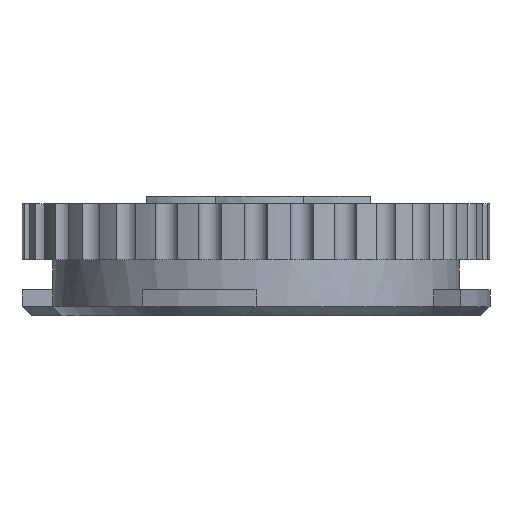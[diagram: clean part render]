
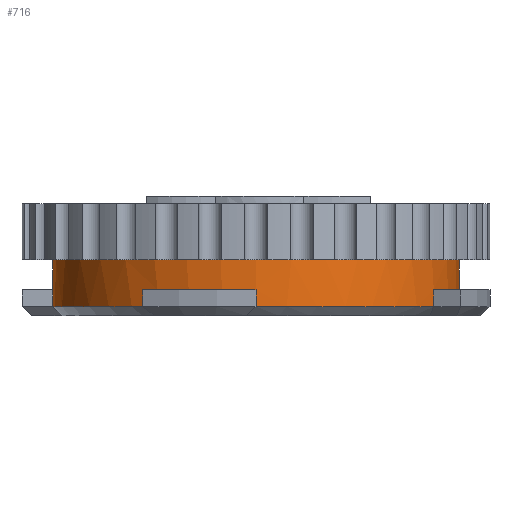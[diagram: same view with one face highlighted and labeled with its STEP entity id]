
A CAD part, front view. The second image highlights one B-rep face of the part: STEP entity #716.
In plain terms, the highlighted cylindrical face has radius 13.787 mm (diameter 27.575 mm), a partial arc.
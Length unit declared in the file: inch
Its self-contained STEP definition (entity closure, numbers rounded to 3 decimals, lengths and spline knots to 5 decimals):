
#70 = VECTOR ( 'NONE', #9266, 39.37008 ) ;
#74 = CARTESIAN_POINT ( 'NONE',  ( -0.26316, -0.47476, 0.15 ) ) ;
#172 = DIRECTION ( 'NONE',  ( 0., 0., 1. ) ) ;
#273 = EDGE_CURVE ( 'NONE', #2922, #9661, #8090, .T. ) ;
#299 = EDGE_CURVE ( 'NONE', #7053, #6835, #10244, .T. ) ;
#336 = VECTOR ( 'NONE', #3346, 39.37008 ) ;
#481 = VERTEX_POINT ( 'NONE', #3257 ) ;
#513 = LINE ( 'NONE', #5966, #7070 ) ;
#571 = DIRECTION ( 'NONE',  ( 0., 0., 1. ) ) ;
#663 = CARTESIAN_POINT ( 'NONE',  ( 0., -0.54281, 0.02461 ) ) ;
#678 = FACE_OUTER_BOUND ( 'NONE', #6350, .T. ) ;
#716 = ADVANCED_FACE ( 'NONE', ( #678 ), #5493, .T. ) ;
#2026 = DIRECTION ( 'NONE',  ( 1., 0., 0. ) ) ;
#2131 = EDGE_CURVE ( 'NONE', #2906, #481, #11769, .T. ) ;
#2173 = EDGE_CURVE ( 'NONE', #5177, #5873, #8342, .T. ) ;
#2304 = DIRECTION ( 'NONE',  ( 0., 0., -1. ) ) ;
#2452 = VECTOR ( 'NONE', #10574, 39.37008 ) ;
#2470 = AXIS2_PLACEMENT_3D ( 'NONE', #10222, #7526, #8386 ) ;
#2478 = CARTESIAN_POINT ( 'NONE',  ( -0.54281, 0., 0.15 ) ) ;
#2486 = ORIENTED_EDGE ( 'NONE', *, *, #6301, .T. ) ;
#2507 = LINE ( 'NONE', #7438, #70 ) ;
#2511 = DIRECTION ( 'NONE',  ( 0., 0., 1. ) ) ;
#2636 = DIRECTION ( 'NONE',  ( 1., 0., 0. ) ) ;
#2906 = VERTEX_POINT ( 'NONE', #7974 ) ;
#2922 = VERTEX_POINT ( 'NONE', #2478 ) ;
#3010 = ORIENTED_EDGE ( 'NONE', *, *, #2173, .T. ) ;
#3013 = AXIS2_PLACEMENT_3D ( 'NONE', #8129, #6281, #2636 ) ;
#3239 = DIRECTION ( 'NONE',  ( 0., 0., 1. ) ) ;
#3257 = CARTESIAN_POINT ( 'NONE',  ( 0.54281, 0., 0.07 ) ) ;
#3346 = DIRECTION ( 'NONE',  ( 0., 0., -1. ) ) ;
#3484 = ORIENTED_EDGE ( 'NONE', *, *, #3517, .T. ) ;
#3517 = EDGE_CURVE ( 'NONE', #4905, #8019, #4777, .T. ) ;
#4618 = VECTOR ( 'NONE', #8331, 39.37008 ) ;
#4669 = CARTESIAN_POINT ( 'NONE',  ( 0., 0., 0.02461 ) ) ;
#4703 = DIRECTION ( 'NONE',  ( 0., 0., 1. ) ) ;
#4777 = CIRCLE ( 'NONE', #10552, 0.54281 ) ;
#4895 = LINE ( 'NONE', #74, #4618 ) ;
#4905 = VERTEX_POINT ( 'NONE', #11013 ) ;
#4997 = CARTESIAN_POINT ( 'NONE',  ( -0.54281, 0., 0.07 ) ) ;
#5053 = ORIENTED_EDGE ( 'NONE', *, *, #2131, .T. ) ;
#5093 = AXIS2_PLACEMENT_3D ( 'NONE', #9756, #571, #7854 ) ;
#5177 = VERTEX_POINT ( 'NONE', #4997 ) ;
#5230 = EDGE_CURVE ( 'NONE', #6835, #2906, #513, .T. ) ;
#5493 = CYLINDRICAL_SURFACE ( 'NONE', #2470, 0.54281 ) ;
#5568 = EDGE_CURVE ( 'NONE', #5873, #7610, #11511, .T. ) ;
#5571 = AXIS2_PLACEMENT_3D ( 'NONE', #11255, #4703, #9412 ) ;
#5873 = VERTEX_POINT ( 'NONE', #7384 ) ;
#5943 = CARTESIAN_POINT ( 'NONE',  ( -0.54281, 0., 0.15 ) ) ;
#5960 = CARTESIAN_POINT ( 'NONE',  ( -0.54281, 0., 0.15 ) ) ;
#5966 = CARTESIAN_POINT ( 'NONE',  ( 0.47476, -0.26316, 0.15 ) ) ;
#5986 = CARTESIAN_POINT ( 'NONE',  ( 0., -0.54281, 0.15 ) ) ;
#6079 = CARTESIAN_POINT ( 'NONE',  ( 0., -0.54281, 0.07 ) ) ;
#6095 = ORIENTED_EDGE ( 'NONE', *, *, #7781, .T. ) ;
#6116 = DIRECTION ( 'NONE',  ( 0., -1., 0. ) ) ;
#6281 = DIRECTION ( 'NONE',  ( 0., 0., 1. ) ) ;
#6301 = EDGE_CURVE ( 'NONE', #8019, #7053, #8936, .T. ) ;
#6350 = EDGE_LOOP ( 'NONE', ( #11126, #9489, #6923, #3010, #8493, #6095, #3484, #2486, #10954, #7155, #5053 ) ) ;
#6835 = VERTEX_POINT ( 'NONE', #10700 ) ;
#6923 = ORIENTED_EDGE ( 'NONE', *, *, #9503, .T. ) ;
#7053 = VERTEX_POINT ( 'NONE', #663 ) ;
#7070 = VECTOR ( 'NONE', #3239, 39.37008 ) ;
#7155 = ORIENTED_EDGE ( 'NONE', *, *, #5230, .T. ) ;
#7248 = CARTESIAN_POINT ( 'NONE',  ( -0.26316, -0.47476, 0.02461 ) ) ;
#7297 = LINE ( 'NONE', #5943, #2452 ) ;
#7384 = CARTESIAN_POINT ( 'NONE',  ( -0.54281, 0., 0.02461 ) ) ;
#7438 = CARTESIAN_POINT ( 'NONE',  ( 0.54281, 0., 0.15 ) ) ;
#7526 = DIRECTION ( 'NONE',  ( 0., 0., -1. ) ) ;
#7610 = VERTEX_POINT ( 'NONE', #7248 ) ;
#7624 = VECTOR ( 'NONE', #2304, 39.37008 ) ;
#7781 = EDGE_CURVE ( 'NONE', #7610, #4905, #4895, .T. ) ;
#7824 = EDGE_CURVE ( 'NONE', #9661, #481, #2507, .T. ) ;
#7854 = DIRECTION ( 'NONE',  ( 1., 0., 0. ) ) ;
#7974 = CARTESIAN_POINT ( 'NONE',  ( 0.47476, -0.26316, 0.07 ) ) ;
#8019 = VERTEX_POINT ( 'NONE', #6079 ) ;
#8090 = CIRCLE ( 'NONE', #5571, 0.54281 ) ;
#8129 = CARTESIAN_POINT ( 'NONE',  ( 0., 0., 0.07 ) ) ;
#8331 = DIRECTION ( 'NONE',  ( 0., 0., 1. ) ) ;
#8342 = LINE ( 'NONE', #5960, #336 ) ;
#8386 = DIRECTION ( 'NONE',  ( -1., 0., 0. ) ) ;
#8493 = ORIENTED_EDGE ( 'NONE', *, *, #5568, .T. ) ;
#8936 = LINE ( 'NONE', #5986, #7624 ) ;
#9052 = AXIS2_PLACEMENT_3D ( 'NONE', #4669, #172, #2026 ) ;
#9266 = DIRECTION ( 'NONE',  ( 0., 0., -1. ) ) ;
#9412 = DIRECTION ( 'NONE',  ( 1., 0., 0. ) ) ;
#9489 = ORIENTED_EDGE ( 'NONE', *, *, #273, .F. ) ;
#9503 = EDGE_CURVE ( 'NONE', #2922, #5177, #7297, .T. ) ;
#9661 = VERTEX_POINT ( 'NONE', #11713 ) ;
#9756 = CARTESIAN_POINT ( 'NONE',  ( 0., 0., 0.02461 ) ) ;
#9828 = CARTESIAN_POINT ( 'NONE',  ( 0., 0., 0.07 ) ) ;
#10222 = CARTESIAN_POINT ( 'NONE',  ( 0., 0., 0.15 ) ) ;
#10244 = CIRCLE ( 'NONE', #9052, 0.54281 ) ;
#10552 = AXIS2_PLACEMENT_3D ( 'NONE', #9828, #2511, #6116 ) ;
#10574 = DIRECTION ( 'NONE',  ( 0., 0., -1. ) ) ;
#10700 = CARTESIAN_POINT ( 'NONE',  ( 0.47476, -0.26316, 0.02461 ) ) ;
#10954 = ORIENTED_EDGE ( 'NONE', *, *, #299, .T. ) ;
#11013 = CARTESIAN_POINT ( 'NONE',  ( -0.26316, -0.47476, 0.07 ) ) ;
#11126 = ORIENTED_EDGE ( 'NONE', *, *, #7824, .F. ) ;
#11255 = CARTESIAN_POINT ( 'NONE',  ( 0., 0., 0.15 ) ) ;
#11511 = CIRCLE ( 'NONE', #5093, 0.54281 ) ;
#11713 = CARTESIAN_POINT ( 'NONE',  ( 0.54281, 0., 0.15 ) ) ;
#11769 = CIRCLE ( 'NONE', #3013, 0.54281 ) ;
